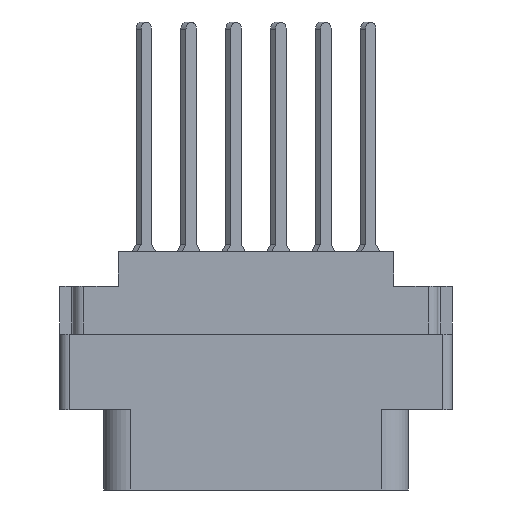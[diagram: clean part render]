
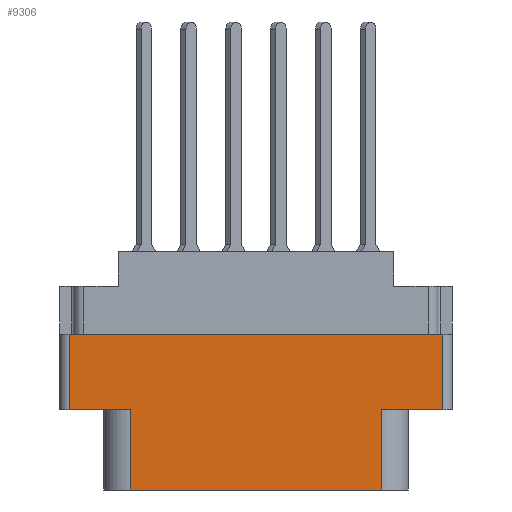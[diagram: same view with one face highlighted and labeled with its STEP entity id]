
A CAD part, front view. The second image highlights one B-rep face of the part: STEP entity #9306.
In plain terms, the highlighted planar face has unit normal (0, -1, 0).
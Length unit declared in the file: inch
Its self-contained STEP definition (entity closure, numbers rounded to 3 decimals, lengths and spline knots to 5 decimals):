
#339 = VERTEX_POINT ( 'NONE', #2038 ) ;
#513 = CARTESIAN_POINT ( 'NONE',  ( -0.624, -0.343, -0.798 ) ) ;
#668 = EDGE_CURVE ( 'NONE', #4103, #18728, #4758, .T. ) ;
#1032 = CARTESIAN_POINT ( 'NONE',  ( -0.42, -0.343, -0.798 ) ) ;
#1277 = FACE_OUTER_BOUND ( 'NONE', #1727, .T. ) ;
#1565 = EDGE_CURVE ( 'NONE', #7506, #5859, #8500, .T. ) ;
#1627 = CARTESIAN_POINT ( 'NONE',  ( -0.42, -0.343, -0.529 ) ) ;
#1683 = LINE ( 'NONE', #2113, #4679 ) ;
#1727 = EDGE_LOOP ( 'NONE', ( #6552, #7676, #9536, #7292, #11063, #13610, #14071, #5452 ) ) ;
#2038 = CARTESIAN_POINT ( 'NONE',  ( 0.624, -0.343, -0.277 ) ) ;
#2113 = CARTESIAN_POINT ( 'NONE',  ( -0.624, -0.343, -0.798 ) ) ;
#2358 = VECTOR ( 'NONE', #5302, 39.37008 ) ;
#2562 = VERTEX_POINT ( 'NONE', #6899 ) ;
#2931 = CARTESIAN_POINT ( 'NONE',  ( 0.42, -0.343, -0.529 ) ) ;
#3445 = VECTOR ( 'NONE', #17672, 39.37008 ) ;
#3570 = VECTOR ( 'NONE', #12275, 39.37008 ) ;
#3989 = LINE ( 'NONE', #4265, #4456 ) ;
#4103 = VERTEX_POINT ( 'NONE', #19448 ) ;
#4265 = CARTESIAN_POINT ( 'NONE',  ( 0., -0.343, -0.529 ) ) ;
#4456 = VECTOR ( 'NONE', #14857, 39.37008 ) ;
#4670 = EDGE_CURVE ( 'NONE', #13560, #19163, #18091, .T. ) ;
#4679 = VECTOR ( 'NONE', #18958, 39.37008 ) ;
#4758 = LINE ( 'NONE', #1627, #3570 ) ;
#5003 = LINE ( 'NONE', #8972, #14559 ) ;
#5302 = DIRECTION ( 'NONE',  ( 0., 0., -1. ) ) ;
#5452 = ORIENTED_EDGE ( 'NONE', *, *, #12864, .T. ) ;
#5859 = VERTEX_POINT ( 'NONE', #2931 ) ;
#6552 = ORIENTED_EDGE ( 'NONE', *, *, #668, .T. ) ;
#6899 = CARTESIAN_POINT ( 'NONE',  ( 0.42, -0.343, -0.798 ) ) ;
#7292 = ORIENTED_EDGE ( 'NONE', *, *, #1565, .F. ) ;
#7506 = VERTEX_POINT ( 'NONE', #9690 ) ;
#7676 = ORIENTED_EDGE ( 'NONE', *, *, #14626, .T. ) ;
#8500 = LINE ( 'NONE', #13327, #3445 ) ;
#8972 = CARTESIAN_POINT ( 'NONE',  ( 0.624, -0.343, -0.798 ) ) ;
#9306 = ADVANCED_FACE ( 'NONE', ( #1277 ), #12640, .T. ) ;
#9536 = ORIENTED_EDGE ( 'NONE', *, *, #12398, .F. ) ;
#9690 = CARTESIAN_POINT ( 'NONE',  ( 0.624, -0.343, -0.529 ) ) ;
#9899 = CARTESIAN_POINT ( 'NONE',  ( 0.42, -0.343, -0.529 ) ) ;
#10020 = DIRECTION ( 'NONE',  ( 0., 0., -1. ) ) ;
#10130 = EDGE_CURVE ( 'NONE', #7506, #339, #5003, .T. ) ;
#11063 = ORIENTED_EDGE ( 'NONE', *, *, #10130, .T. ) ;
#11285 = AXIS2_PLACEMENT_3D ( 'NONE', #513, #14697, #10020 ) ;
#11911 = LINE ( 'NONE', #9899, #2358 ) ;
#12030 = CARTESIAN_POINT ( 'NONE',  ( -0.624, -0.343, -0.277 ) ) ;
#12275 = DIRECTION ( 'NONE',  ( 0., 0., -1. ) ) ;
#12398 = EDGE_CURVE ( 'NONE', #5859, #2562, #11911, .T. ) ;
#12597 = CARTESIAN_POINT ( 'NONE',  ( -0.656, -0.343, -0.277 ) ) ;
#12640 = PLANE ( 'NONE',  #11285 ) ;
#12864 = EDGE_CURVE ( 'NONE', #13560, #4103, #3989, .T. ) ;
#13071 = VECTOR ( 'NONE', #13293, 39.37008 ) ;
#13185 = EDGE_CURVE ( 'NONE', #19163, #339, #16133, .T. ) ;
#13259 = VECTOR ( 'NONE', #15668, 39.37008 ) ;
#13293 = DIRECTION ( 'NONE',  ( 0., 0., 1. ) ) ;
#13327 = CARTESIAN_POINT ( 'NONE',  ( 0., -0.343, -0.529 ) ) ;
#13560 = VERTEX_POINT ( 'NONE', #16203 ) ;
#13610 = ORIENTED_EDGE ( 'NONE', *, *, #13185, .F. ) ;
#14071 = ORIENTED_EDGE ( 'NONE', *, *, #4670, .F. ) ;
#14559 = VECTOR ( 'NONE', #19563, 39.37008 ) ;
#14626 = EDGE_CURVE ( 'NONE', #18728, #2562, #1683, .T. ) ;
#14697 = DIRECTION ( 'NONE',  ( 0., -1., 0. ) ) ;
#14762 = CARTESIAN_POINT ( 'NONE',  ( -0.624, -0.343, -0.798 ) ) ;
#14857 = DIRECTION ( 'NONE',  ( 1., 0., 0. ) ) ;
#15668 = DIRECTION ( 'NONE',  ( 1., 0., 0. ) ) ;
#16133 = LINE ( 'NONE', #12597, #13259 ) ;
#16203 = CARTESIAN_POINT ( 'NONE',  ( -0.624, -0.343, -0.529 ) ) ;
#17672 = DIRECTION ( 'NONE',  ( -1., 0., 0. ) ) ;
#18091 = LINE ( 'NONE', #14762, #13071 ) ;
#18728 = VERTEX_POINT ( 'NONE', #1032 ) ;
#18958 = DIRECTION ( 'NONE',  ( 1., 0., 0. ) ) ;
#19163 = VERTEX_POINT ( 'NONE', #12030 ) ;
#19448 = CARTESIAN_POINT ( 'NONE',  ( -0.42, -0.343, -0.529 ) ) ;
#19563 = DIRECTION ( 'NONE',  ( 0., 0., 1. ) ) ;
